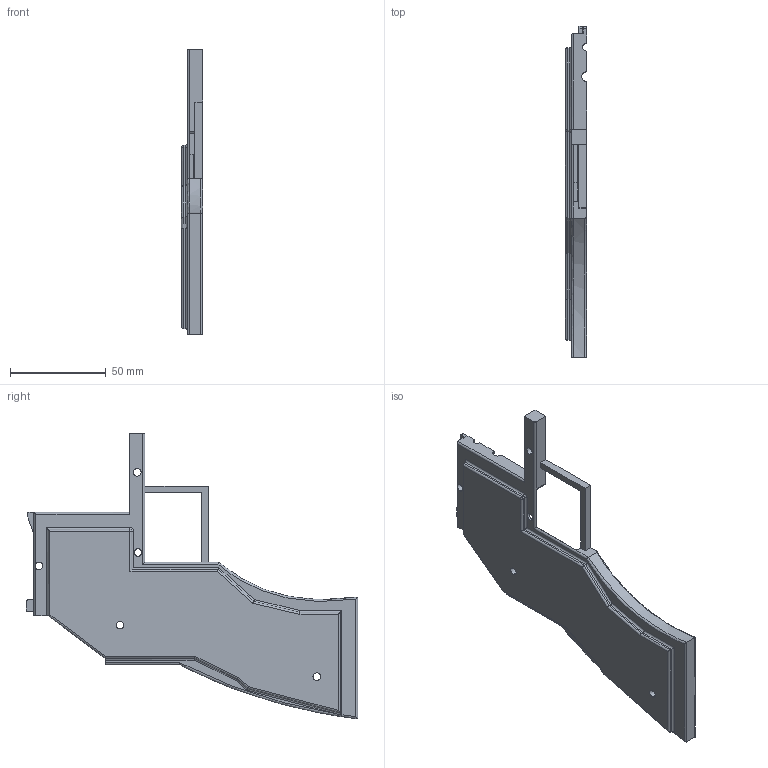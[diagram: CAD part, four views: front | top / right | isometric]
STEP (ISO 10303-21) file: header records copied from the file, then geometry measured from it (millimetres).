
FILE_DESCRIPTION (( 'STEP AP203' ), '1' );
FILE_NAME ('frame_half_R.STEP', '2013-08-18T03:46:27', ( '' ), ( '' ), 'SwSTEP 2.0', 'SolidWorks 2012', '' );
FILE_SCHEMA (( 'CONFIG_CONTROL_DESIGN' ));
Length unit declared in the file: millimetre
Products named in the file (1): frame_half_R
Bounding box: 11 x 173.54 x 149.61 mm (x, y, z)
Volume: 72511.6 mm3; surface area: 30994.3 mm2
Topology: 1 solids, 1 shells, 209 faces, 561 edges, 348 vertices
Faces by surface type: plane 109, cylinder 79, bspline 12, torus 6, sphere 3
Entity records: 7110 total; most frequent: CARTESIAN_POINT 2004, ORIENTED_EDGE 1116, DIRECTION 966, EDGE_CURVE 558, LINE 386, VECTOR 386, VERTEX_POINT 348, AXIS2_PLACEMENT_3D 290
